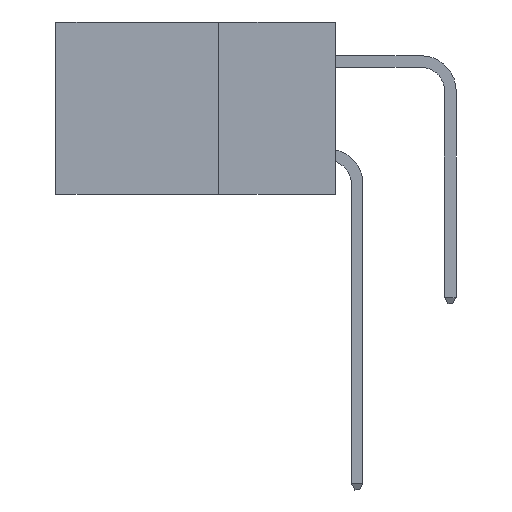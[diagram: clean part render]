
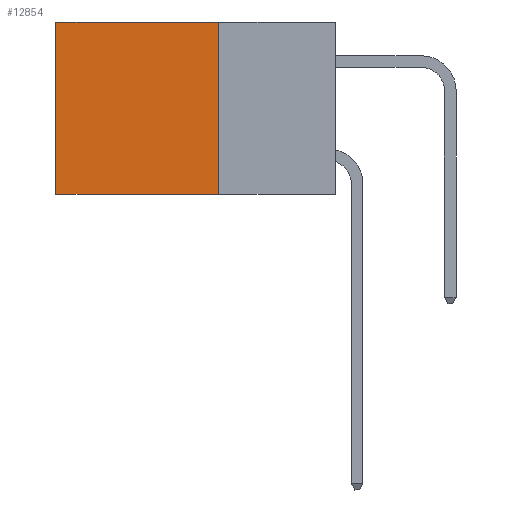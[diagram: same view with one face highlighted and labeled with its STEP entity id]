
A CAD part, left-side view. The second image highlights one B-rep face of the part: STEP entity #12854.
In plain terms, the highlighted planar face has unit normal (-1, 0, 0).
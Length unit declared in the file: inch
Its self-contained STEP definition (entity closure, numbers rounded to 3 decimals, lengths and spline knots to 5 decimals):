
#1123 = EDGE_LOOP ( 'NONE', ( #6763, #18741, #5254, #15740 ) ) ;
#1374 = VERTEX_POINT ( 'NONE', #15745 ) ;
#1440 = CARTESIAN_POINT ( 'NONE',  ( 0.2875, 0.25, 0. ) ) ;
#1944 = CARTESIAN_POINT ( 'NONE',  ( 0.2875, 0.25, 0. ) ) ;
#2068 = DIRECTION ( 'NONE',  ( 0., 0., -1. ) ) ;
#2956 = LINE ( 'NONE', #16799, #11389 ) ;
#3154 = VECTOR ( 'NONE', #2068, 39.37008 ) ;
#3566 = EDGE_CURVE ( 'NONE', #20367, #14277, #2956, .T. ) ;
#3796 = DIRECTION ( 'NONE',  ( 0., 0., -1. ) ) ;
#4480 = DIRECTION ( 'NONE',  ( 0., 1., 0. ) ) ;
#4530 = VECTOR ( 'NONE', #4480, 39.37008 ) ;
#4874 = CARTESIAN_POINT ( 'NONE',  ( 0.2875, 0.25, 0. ) ) ;
#5254 = ORIENTED_EDGE ( 'NONE', *, *, #13850, .F. ) ;
#5569 = EDGE_CURVE ( 'NONE', #14277, #12180, #7993, .T. ) ;
#5792 = FACE_OUTER_BOUND ( 'NONE', #1123, .T. ) ;
#6763 = ORIENTED_EDGE ( 'NONE', *, *, #5569, .T. ) ;
#7993 = LINE ( 'NONE', #12836, #3154 ) ;
#8962 = CARTESIAN_POINT ( 'NONE',  ( 0.2875, 0.6, 0. ) ) ;
#9037 = EDGE_CURVE ( 'NONE', #1374, #12180, #9860, .T. ) ;
#9548 = AXIS2_PLACEMENT_3D ( 'NONE', #1944, #14478, #3796 ) ;
#9860 = LINE ( 'NONE', #18659, #4530 ) ;
#11389 = VECTOR ( 'NONE', #11493, 39.37008 ) ;
#11493 = DIRECTION ( 'NONE',  ( 0., 1., 0. ) ) ;
#12180 = VERTEX_POINT ( 'NONE', #14370 ) ;
#12836 = CARTESIAN_POINT ( 'NONE',  ( 0.2875, 0.6, 0. ) ) ;
#12854 = ADVANCED_FACE ( 'NONE', ( #5792 ), #21408, .F. ) ;
#13364 = VECTOR ( 'NONE', #19270, 39.37008 ) ;
#13850 = EDGE_CURVE ( 'NONE', #20367, #1374, #17537, .T. ) ;
#14277 = VERTEX_POINT ( 'NONE', #8962 ) ;
#14370 = CARTESIAN_POINT ( 'NONE',  ( 0.2875, 0.6, -0.37 ) ) ;
#14478 = DIRECTION ( 'NONE',  ( 1., 0., 0. ) ) ;
#15740 = ORIENTED_EDGE ( 'NONE', *, *, #3566, .T. ) ;
#15745 = CARTESIAN_POINT ( 'NONE',  ( 0.2875, 0.25, -0.37 ) ) ;
#16799 = CARTESIAN_POINT ( 'NONE',  ( 0.2875, 0.25, 0. ) ) ;
#17537 = LINE ( 'NONE', #1440, #13364 ) ;
#18659 = CARTESIAN_POINT ( 'NONE',  ( 0.2875, 0.25, -0.37 ) ) ;
#18741 = ORIENTED_EDGE ( 'NONE', *, *, #9037, .F. ) ;
#19270 = DIRECTION ( 'NONE',  ( 0., 0., -1. ) ) ;
#20367 = VERTEX_POINT ( 'NONE', #4874 ) ;
#21408 = PLANE ( 'NONE',  #9548 ) ;
